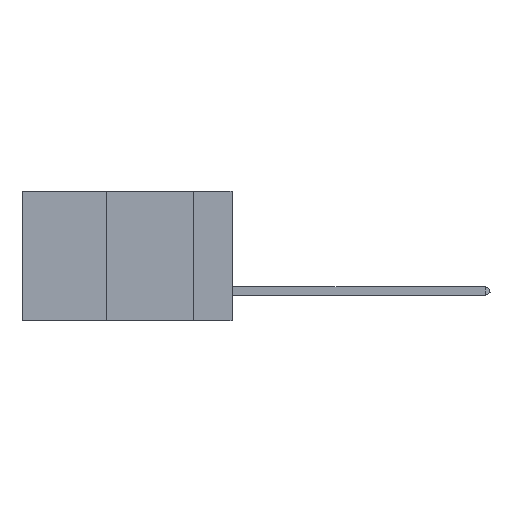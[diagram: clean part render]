
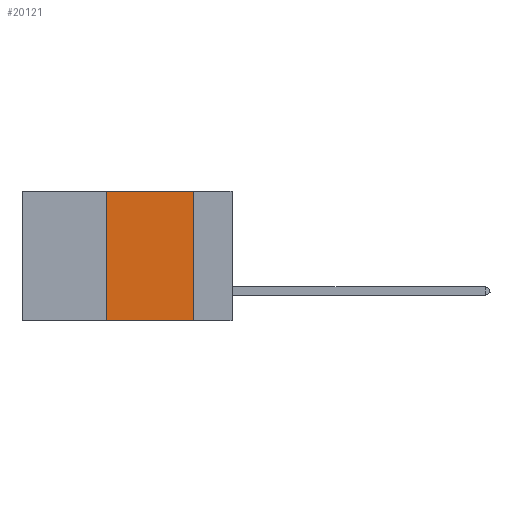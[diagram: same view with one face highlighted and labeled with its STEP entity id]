
A CAD part, left-side view. The second image highlights one B-rep face of the part: STEP entity #20121.
In plain terms, the highlighted planar face has unit normal (-1, 0, 0).
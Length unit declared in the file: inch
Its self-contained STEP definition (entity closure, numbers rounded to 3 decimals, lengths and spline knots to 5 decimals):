
#208 = CARTESIAN_POINT ( 'NONE',  ( 0., 0.6, 0. ) ) ;
#2458 = LINE ( 'NONE', #15352, #29482 ) ;
#4566 = EDGE_CURVE ( 'NONE', #11167, #6821, #13587, .T. ) ;
#5573 = CARTESIAN_POINT ( 'NONE',  ( 0., 0.36, 0. ) ) ;
#6821 = VERTEX_POINT ( 'NONE', #31295 ) ;
#9731 = DIRECTION ( 'NONE',  ( 0., 0., -1. ) ) ;
#9923 = LINE ( 'NONE', #14495, #16070 ) ;
#11144 = DIRECTION ( 'NONE',  ( 0., -1., 0. ) ) ;
#11167 = VERTEX_POINT ( 'NONE', #28411 ) ;
#12540 = CARTESIAN_POINT ( 'NONE',  ( 0., 0.11, -0.37 ) ) ;
#13318 = CARTESIAN_POINT ( 'NONE',  ( 0., 0.6, -0.37 ) ) ;
#13587 = LINE ( 'NONE', #5573, #45552 ) ;
#13932 = ORIENTED_EDGE ( 'NONE', *, *, #43461, .F. ) ;
#14042 = CARTESIAN_POINT ( 'NONE',  ( 0., 0.11, 0. ) ) ;
#14495 = CARTESIAN_POINT ( 'NONE',  ( 0., 0.11, 0. ) ) ;
#15352 = CARTESIAN_POINT ( 'NONE',  ( 0., 0.6, 0. ) ) ;
#15962 = DIRECTION ( 'NONE',  ( 0., 0., 1. ) ) ;
#16070 = VECTOR ( 'NONE', #42522, 39.37008 ) ;
#20121 = ADVANCED_FACE ( 'NONE', ( #26484 ), #44866, .F. ) ;
#21350 = EDGE_CURVE ( 'NONE', #11167, #26222, #41385, .T. ) ;
#24162 = ORIENTED_EDGE ( 'NONE', *, *, #4566, .F. ) ;
#24238 = AXIS2_PLACEMENT_3D ( 'NONE', #208, #36384, #9731 ) ;
#26222 = VERTEX_POINT ( 'NONE', #12540 ) ;
#26484 = FACE_OUTER_BOUND ( 'NONE', #34332, .T. ) ;
#26994 = VERTEX_POINT ( 'NONE', #14042 ) ;
#27031 = VECTOR ( 'NONE', #41517, 39.37008 ) ;
#28411 = CARTESIAN_POINT ( 'NONE',  ( 0., 0.36, -0.37 ) ) ;
#28617 = ORIENTED_EDGE ( 'NONE', *, *, #33878, .F. ) ;
#29482 = VECTOR ( 'NONE', #11144, 39.37008 ) ;
#31295 = CARTESIAN_POINT ( 'NONE',  ( 0., 0.36, 0. ) ) ;
#33878 = EDGE_CURVE ( 'NONE', #26994, #26222, #9923, .T. ) ;
#34332 = EDGE_LOOP ( 'NONE', ( #28617, #13932, #24162, #44836 ) ) ;
#36384 = DIRECTION ( 'NONE',  ( 1., 0., 0. ) ) ;
#41385 = LINE ( 'NONE', #13318, #27031 ) ;
#41517 = DIRECTION ( 'NONE',  ( 0., -1., 0. ) ) ;
#42522 = DIRECTION ( 'NONE',  ( 0., 0., -1. ) ) ;
#43461 = EDGE_CURVE ( 'NONE', #6821, #26994, #2458, .T. ) ;
#44836 = ORIENTED_EDGE ( 'NONE', *, *, #21350, .T. ) ;
#44866 = PLANE ( 'NONE',  #24238 ) ;
#45552 = VECTOR ( 'NONE', #15962, 39.37008 ) ;
